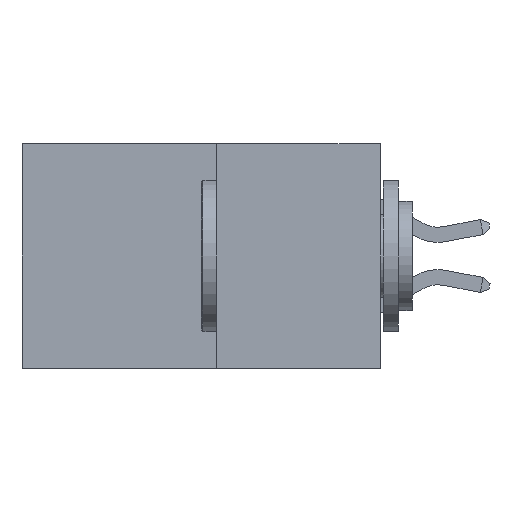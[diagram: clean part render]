
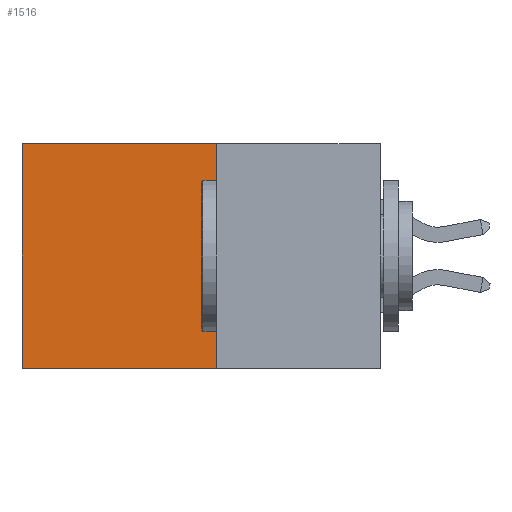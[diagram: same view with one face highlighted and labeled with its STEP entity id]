
A CAD part, left-side view. The second image highlights one B-rep face of the part: STEP entity #1516.
In plain terms, the highlighted planar face has unit normal (-1, 0, 0).
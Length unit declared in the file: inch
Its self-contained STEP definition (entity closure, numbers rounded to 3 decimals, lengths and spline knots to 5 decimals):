
#209 = EDGE_CURVE ( 'NONE', #3855, #14924, #12512, .T. ) ;
#914 = EDGE_CURVE ( 'NONE', #8315, #13223, #3335, .T. ) ;
#1453 = FACE_OUTER_BOUND ( 'NONE', #9157, .T. ) ;
#1516 = ADVANCED_FACE ( 'NONE', ( #1453 ), #10055, .F. ) ;
#3335 = LINE ( 'NONE', #6776, #9360 ) ;
#3376 = CARTESIAN_POINT ( 'NONE',  ( 0.277, 0.27, 0. ) ) ;
#3672 = VECTOR ( 'NONE', #12535, 39.37008 ) ;
#3784 = DIRECTION ( 'NONE',  ( 0., 1., 0. ) ) ;
#3855 = VERTEX_POINT ( 'NONE', #4166 ) ;
#4166 = CARTESIAN_POINT ( 'NONE',  ( 0.277, 0.27, -0.37 ) ) ;
#4478 = EDGE_CURVE ( 'NONE', #13223, #14924, #5236, .T. ) ;
#4538 = CARTESIAN_POINT ( 'NONE',  ( 0.277, 0.27, -0.37 ) ) ;
#5177 = CARTESIAN_POINT ( 'NONE',  ( 0.277, 0.59, 0. ) ) ;
#5236 = LINE ( 'NONE', #13960, #11292 ) ;
#5288 = ORIENTED_EDGE ( 'NONE', *, *, #4478, .T. ) ;
#5668 = ORIENTED_EDGE ( 'NONE', *, *, #914, .T. ) ;
#6776 = CARTESIAN_POINT ( 'NONE',  ( 0.277, 0.27, 0. ) ) ;
#7185 = DIRECTION ( 'NONE',  ( 0., 0., -1. ) ) ;
#7199 = LINE ( 'NONE', #14875, #3672 ) ;
#8315 = VERTEX_POINT ( 'NONE', #3376 ) ;
#8505 = ORIENTED_EDGE ( 'NONE', *, *, #209, .F. ) ;
#9157 = EDGE_LOOP ( 'NONE', ( #5288, #8505, #11717, #5668 ) ) ;
#9358 = VECTOR ( 'NONE', #3784, 39.37008 ) ;
#9360 = VECTOR ( 'NONE', #14306, 39.37008 ) ;
#9393 = DIRECTION ( 'NONE',  ( 0., 0., -1. ) ) ;
#9774 = DIRECTION ( 'NONE',  ( 1., 0., 0. ) ) ;
#10055 = PLANE ( 'NONE',  #11707 ) ;
#10393 = CARTESIAN_POINT ( 'NONE',  ( 0.277, 0.59, -0.37 ) ) ;
#11292 = VECTOR ( 'NONE', #9393, 39.37008 ) ;
#11707 = AXIS2_PLACEMENT_3D ( 'NONE', #13439, #9774, #7185 ) ;
#11717 = ORIENTED_EDGE ( 'NONE', *, *, #13306, .F. ) ;
#12512 = LINE ( 'NONE', #4538, #9358 ) ;
#12535 = DIRECTION ( 'NONE',  ( 0., 0., -1. ) ) ;
#13223 = VERTEX_POINT ( 'NONE', #5177 ) ;
#13306 = EDGE_CURVE ( 'NONE', #8315, #3855, #7199, .T. ) ;
#13439 = CARTESIAN_POINT ( 'NONE',  ( 0.277, 0.27, -0.37 ) ) ;
#13960 = CARTESIAN_POINT ( 'NONE',  ( 0.277, 0.59, -0.37 ) ) ;
#14306 = DIRECTION ( 'NONE',  ( 0., 1., 0. ) ) ;
#14875 = CARTESIAN_POINT ( 'NONE',  ( 0.277, 0.27, -0.37 ) ) ;
#14924 = VERTEX_POINT ( 'NONE', #10393 ) ;
